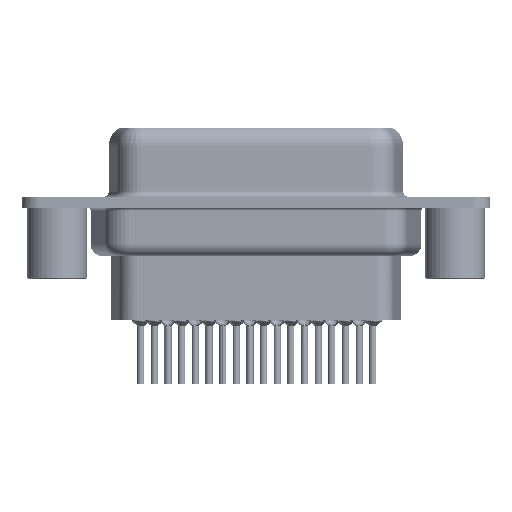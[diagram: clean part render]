
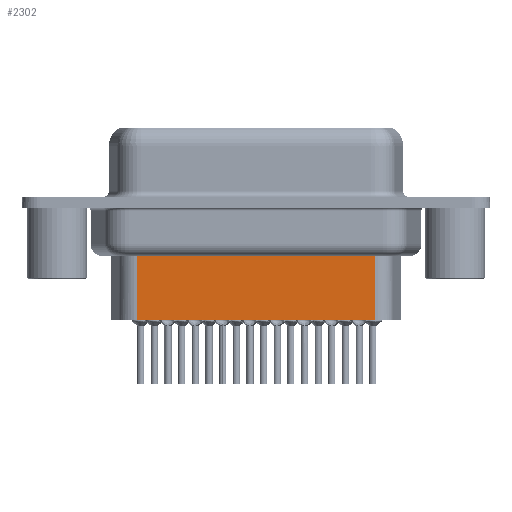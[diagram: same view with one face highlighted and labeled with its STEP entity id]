
A CAD part, front view. The second image highlights one B-rep face of the part: STEP entity #2302.
In plain terms, the highlighted planar face has unit normal (0, -1, 0).
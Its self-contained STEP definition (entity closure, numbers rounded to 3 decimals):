
#905 = CARTESIAN_POINT ( 'NONE',  ( 6.444, -3.5, -4.097 ) ) ;
#2058 = EDGE_CURVE ( 'NONE', #13130, #25393, #30418, .T. ) ;
#2302 = ADVANCED_FACE ( 'NONE', ( #7849 ), #10694, .T. ) ;
#3208 = DIRECTION ( 'NONE',  ( 0., 0., -1. ) ) ;
#3440 = ORIENTED_EDGE ( 'NONE', *, *, #9770, .F. ) ;
#3501 = VECTOR ( 'NONE', #23863, 1000. ) ;
#3537 = ORIENTED_EDGE ( 'NONE', *, *, #15000, .T. ) ;
#4801 = ORIENTED_EDGE ( 'NONE', *, *, #23984, .F. ) ;
#5671 = CARTESIAN_POINT ( 'NONE',  ( 6.691, -3.5, -3.1 ) ) ;
#6194 = CARTESIAN_POINT ( 'NONE',  ( 6.691, -3.5, -9.85 ) ) ;
#6352 = EDGE_LOOP ( 'NONE', ( #4801, #3537, #22530, #3440 ) ) ;
#7849 = FACE_OUTER_BOUND ( 'NONE', #6352, .T. ) ;
#8374 = CARTESIAN_POINT ( 'NONE',  ( 6.691, -3.5, -9.85 ) ) ;
#9770 = EDGE_CURVE ( 'NONE', #23939, #25393, #13914, .T. ) ;
#10694 = PLANE ( 'NONE',  #12915 ) ;
#12915 = AXIS2_PLACEMENT_3D ( 'NONE', #5671, #15918, #21788 ) ;
#13130 = VERTEX_POINT ( 'NONE', #17380 ) ;
#13914 = LINE ( 'NONE', #8374, #3501 ) ;
#14593 = CARTESIAN_POINT ( 'NONE',  ( 6.691, -3.5, -3.1 ) ) ;
#15000 = EDGE_CURVE ( 'NONE', #25681, #13130, #21586, .T. ) ;
#15918 = DIRECTION ( 'NONE',  ( 0., -1., 0. ) ) ;
#17380 = CARTESIAN_POINT ( 'NONE',  ( 6.691, -3.5, -4.097 ) ) ;
#17776 = CARTESIAN_POINT ( 'NONE',  ( 26.629, -3.5, -4.097 ) ) ;
#18520 = LINE ( 'NONE', #19010, #25504 ) ;
#19010 = CARTESIAN_POINT ( 'NONE',  ( 26.629, -3.5, -3.1 ) ) ;
#20059 = VECTOR ( 'NONE', #27733, 1000. ) ;
#21256 = DIRECTION ( 'NONE',  ( -1., 0., 0. ) ) ;
#21531 = CARTESIAN_POINT ( 'NONE',  ( 26.629, -3.5, -9.85 ) ) ;
#21586 = LINE ( 'NONE', #905, #25192 ) ;
#21788 = DIRECTION ( 'NONE',  ( 1., 0., 0. ) ) ;
#22530 = ORIENTED_EDGE ( 'NONE', *, *, #2058, .T. ) ;
#23863 = DIRECTION ( 'NONE',  ( -1., 0., 0. ) ) ;
#23939 = VERTEX_POINT ( 'NONE', #21531 ) ;
#23984 = EDGE_CURVE ( 'NONE', #25681, #23939, #18520, .T. ) ;
#25192 = VECTOR ( 'NONE', #21256, 1000. ) ;
#25393 = VERTEX_POINT ( 'NONE', #6194 ) ;
#25504 = VECTOR ( 'NONE', #3208, 1000. ) ;
#25681 = VERTEX_POINT ( 'NONE', #17776 ) ;
#27733 = DIRECTION ( 'NONE',  ( 0., 0., -1. ) ) ;
#30418 = LINE ( 'NONE', #14593, #20059 ) ;
